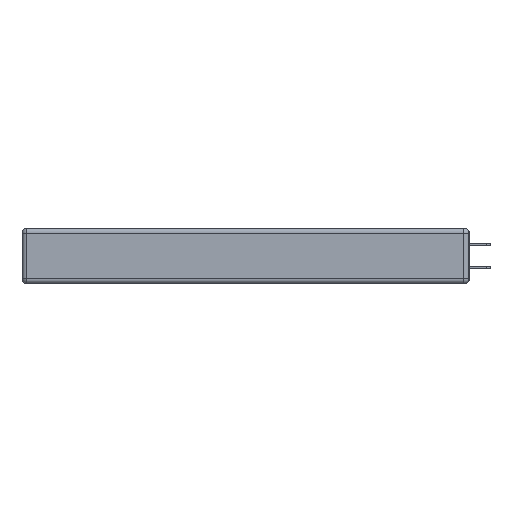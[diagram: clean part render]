
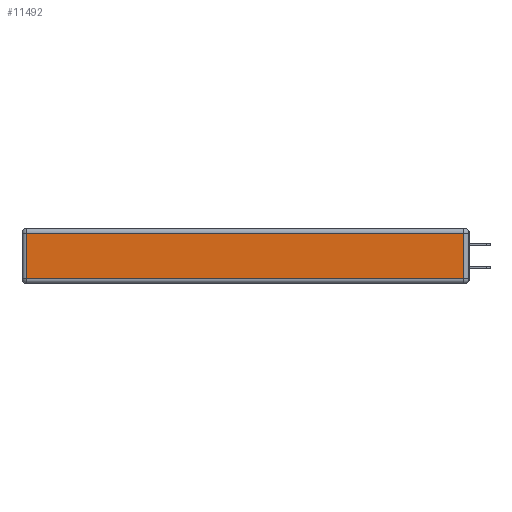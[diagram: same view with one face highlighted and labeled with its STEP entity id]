
A CAD part, left-side view. The second image highlights one B-rep face of the part: STEP entity #11492.
In plain terms, the highlighted planar face has unit normal (-1, 0, 0).
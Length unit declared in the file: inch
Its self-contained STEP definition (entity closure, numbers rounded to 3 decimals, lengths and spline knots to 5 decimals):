
#1124 = LINE ( 'NONE', #23910, #18236 ) ;
#4070 = DIRECTION ( 'NONE',  ( 0., 1., 0. ) ) ;
#5633 = CARTESIAN_POINT ( 'NONE',  ( 0., 0.03, -0.313 ) ) ;
#5920 = VERTEX_POINT ( 'NONE', #10425 ) ;
#6248 = DIRECTION ( 'NONE',  ( 0., -1., 0. ) ) ;
#6335 = LINE ( 'NONE', #19318, #16116 ) ;
#6521 = VERTEX_POINT ( 'NONE', #5633 ) ;
#7475 = AXIS2_PLACEMENT_3D ( 'NONE', #8444, #26312, #17512 ) ;
#8444 = CARTESIAN_POINT ( 'NONE',  ( 0., 0., -0.343 ) ) ;
#8949 = ORIENTED_EDGE ( 'NONE', *, *, #22695, .T. ) ;
#9158 = FACE_OUTER_BOUND ( 'NONE', #28830, .T. ) ;
#10425 = CARTESIAN_POINT ( 'NONE',  ( 0., 0.03, -0.03 ) ) ;
#11492 = ADVANCED_FACE ( 'NONE', ( #9158 ), #22195, .T. ) ;
#11911 = ORIENTED_EDGE ( 'NONE', *, *, #22855, .T. ) ;
#14058 = VECTOR ( 'NONE', #20667, 39.37008 ) ;
#16054 = VECTOR ( 'NONE', #25692, 39.37008 ) ;
#16116 = VECTOR ( 'NONE', #4070, 39.37008 ) ;
#16875 = CARTESIAN_POINT ( 'NONE',  ( 0., 2.72, -0.03 ) ) ;
#17212 = ORIENTED_EDGE ( 'NONE', *, *, #24091, .T. ) ;
#17512 = DIRECTION ( 'NONE',  ( 0., 0., 1. ) ) ;
#18236 = VECTOR ( 'NONE', #6248, 39.37008 ) ;
#18834 = CARTESIAN_POINT ( 'NONE',  ( 0., 2.72, -0.313 ) ) ;
#19318 = CARTESIAN_POINT ( 'NONE',  ( 0., 2.75, -0.03 ) ) ;
#19934 = LINE ( 'NONE', #27598, #14058 ) ;
#19937 = VERTEX_POINT ( 'NONE', #16875 ) ;
#20583 = LINE ( 'NONE', #20743, #16054 ) ;
#20667 = DIRECTION ( 'NONE',  ( 0., 0., 1. ) ) ;
#20743 = CARTESIAN_POINT ( 'NONE',  ( 0., 2.72, -0.343 ) ) ;
#20954 = VERTEX_POINT ( 'NONE', #18834 ) ;
#22195 = PLANE ( 'NONE',  #7475 ) ;
#22695 = EDGE_CURVE ( 'NONE', #20954, #6521, #1124, .T. ) ;
#22855 = EDGE_CURVE ( 'NONE', #5920, #19937, #6335, .T. ) ;
#23910 = CARTESIAN_POINT ( 'NONE',  ( 0., 0., -0.313 ) ) ;
#24091 = EDGE_CURVE ( 'NONE', #19937, #20954, #20583, .T. ) ;
#24407 = EDGE_CURVE ( 'NONE', #6521, #5920, #19934, .T. ) ;
#25692 = DIRECTION ( 'NONE',  ( 0., 0., -1. ) ) ;
#26312 = DIRECTION ( 'NONE',  ( -1., 0., 0. ) ) ;
#27598 = CARTESIAN_POINT ( 'NONE',  ( 0., 0.03, -0.343 ) ) ;
#28130 = ORIENTED_EDGE ( 'NONE', *, *, #24407, .T. ) ;
#28830 = EDGE_LOOP ( 'NONE', ( #8949, #28130, #11911, #17212 ) ) ;
